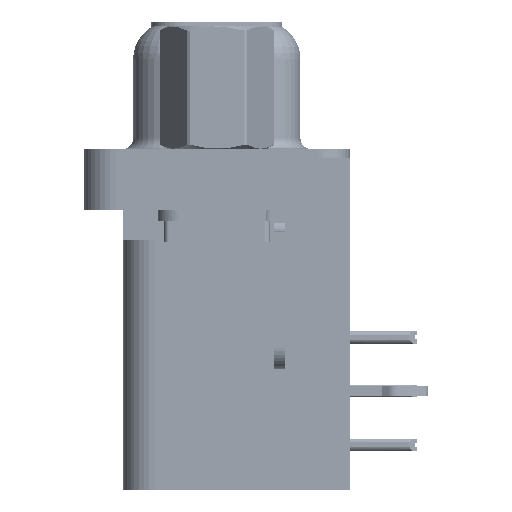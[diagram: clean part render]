
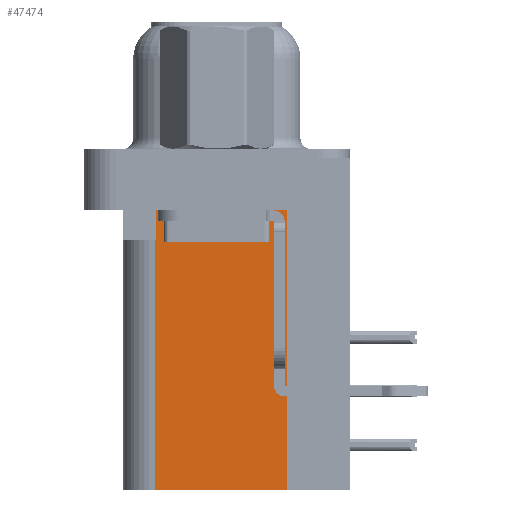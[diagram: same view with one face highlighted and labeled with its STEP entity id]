
A CAD part, left-side view. The second image highlights one B-rep face of the part: STEP entity #47474.
In plain terms, the highlighted planar face has unit normal (-1, 0, 0).
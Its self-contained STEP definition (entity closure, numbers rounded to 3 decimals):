
#296 = LINE ( 'NONE', #12360, #46432 ) ;
#1989 = DIRECTION ( 'NONE',  ( 0., 0., -1. ) ) ;
#2689 = DIRECTION ( 'NONE',  ( 1., 0., 0. ) ) ;
#3903 = DIRECTION ( 'NONE',  ( 0., 0., 1. ) ) ;
#4878 = EDGE_LOOP ( 'NONE', ( #55812, #40858, #33827, #54229, #33194, #53748 ) ) ;
#5639 = CARTESIAN_POINT ( 'NONE',  ( 3.79, 2.895, -2.5 ) ) ;
#11368 = DIRECTION ( 'NONE',  ( 0., 1., 0. ) ) ;
#11500 = CARTESIAN_POINT ( 'NONE',  ( 3.79, -3.295, -15.7 ) ) ;
#12360 = CARTESIAN_POINT ( 'NONE',  ( 3.79, -3.295, -15.7 ) ) ;
#12975 = VECTOR ( 'NONE', #1989, 1000. ) ;
#14525 = FACE_OUTER_BOUND ( 'NONE', #4878, .T. ) ;
#14684 = VECTOR ( 'NONE', #11368, 1000. ) ;
#16575 = DIRECTION ( 'NONE',  ( 0., 0., 1. ) ) ;
#17605 = CARTESIAN_POINT ( 'NONE',  ( 3.79, -3.295, -2.5 ) ) ;
#22051 = DIRECTION ( 'NONE',  ( 0., 1., 0. ) ) ;
#25390 = AXIS2_PLACEMENT_3D ( 'NONE', #11500, #2689, #33852 ) ;
#25710 = VERTEX_POINT ( 'NONE', #34417 ) ;
#26535 = LINE ( 'NONE', #38026, #14684 ) ;
#29342 = CARTESIAN_POINT ( 'NONE',  ( 3.79, -3.295, -15.7 ) ) ;
#29523 = LINE ( 'NONE', #30594, #39999 ) ;
#30327 = EDGE_CURVE ( 'NONE', #54948, #25710, #46124, .T. ) ;
#30594 = CARTESIAN_POINT ( 'NONE',  ( 3.79, -3.295, -15.7 ) ) ;
#30786 = VERTEX_POINT ( 'NONE', #34190 ) ;
#31757 = EDGE_CURVE ( 'NONE', #30786, #55427, #55768, .T. ) ;
#33194 = ORIENTED_EDGE ( 'NONE', *, *, #51649, .F. ) ;
#33350 = VERTEX_POINT ( 'NONE', #55900 ) ;
#33546 = CARTESIAN_POINT ( 'NONE',  ( 3.79, 2.925, -15.7 ) ) ;
#33827 = ORIENTED_EDGE ( 'NONE', *, *, #44893, .T. ) ;
#33852 = DIRECTION ( 'NONE',  ( 0., 0., -1. ) ) ;
#34190 = CARTESIAN_POINT ( 'NONE',  ( 3.79, -3.295, -2.5 ) ) ;
#34417 = CARTESIAN_POINT ( 'NONE',  ( 3.79, 2.925, -3.9 ) ) ;
#37424 = EDGE_CURVE ( 'NONE', #49812, #30786, #29523, .T. ) ;
#38026 = CARTESIAN_POINT ( 'NONE',  ( 3.79, 0., -3.9 ) ) ;
#39999 = VECTOR ( 'NONE', #3903, 1000. ) ;
#40468 = EDGE_CURVE ( 'NONE', #55427, #33350, #48585, .T. ) ;
#40858 = ORIENTED_EDGE ( 'NONE', *, *, #40468, .T. ) ;
#41998 = CARTESIAN_POINT ( 'NONE',  ( 3.79, 2.895, -3.9 ) ) ;
#43595 = DIRECTION ( 'NONE',  ( 0., 1., 0. ) ) ;
#44893 = EDGE_CURVE ( 'NONE', #33350, #25710, #26535, .T. ) ;
#46124 = LINE ( 'NONE', #52313, #56601 ) ;
#46432 = VECTOR ( 'NONE', #43595, 1000. ) ;
#47221 = PLANE ( 'NONE',  #25390 ) ;
#47474 = ADVANCED_FACE ( 'NONE', ( #14525 ), #47221, .F. ) ;
#48585 = LINE ( 'NONE', #41998, #12975 ) ;
#49812 = VERTEX_POINT ( 'NONE', #29342 ) ;
#51649 = EDGE_CURVE ( 'NONE', #49812, #54948, #296, .T. ) ;
#52313 = CARTESIAN_POINT ( 'NONE',  ( 3.79, 2.925, -15.7 ) ) ;
#52958 = VECTOR ( 'NONE', #22051, 1000. ) ;
#53748 = ORIENTED_EDGE ( 'NONE', *, *, #37424, .T. ) ;
#54229 = ORIENTED_EDGE ( 'NONE', *, *, #30327, .F. ) ;
#54948 = VERTEX_POINT ( 'NONE', #33546 ) ;
#55427 = VERTEX_POINT ( 'NONE', #5639 ) ;
#55768 = LINE ( 'NONE', #17605, #52958 ) ;
#55812 = ORIENTED_EDGE ( 'NONE', *, *, #31757, .T. ) ;
#55900 = CARTESIAN_POINT ( 'NONE',  ( 3.79, 2.895, -3.9 ) ) ;
#56601 = VECTOR ( 'NONE', #16575, 1000. ) ;
